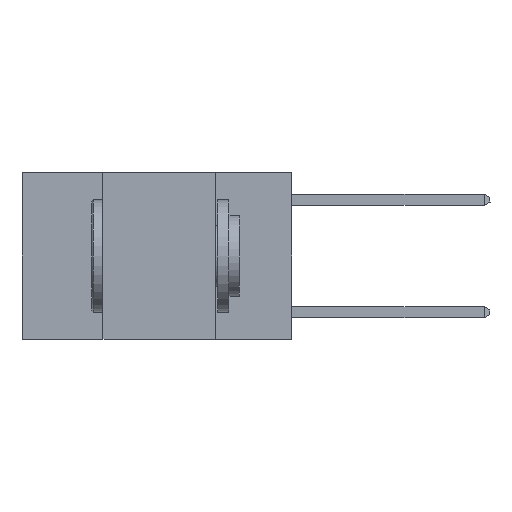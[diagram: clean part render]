
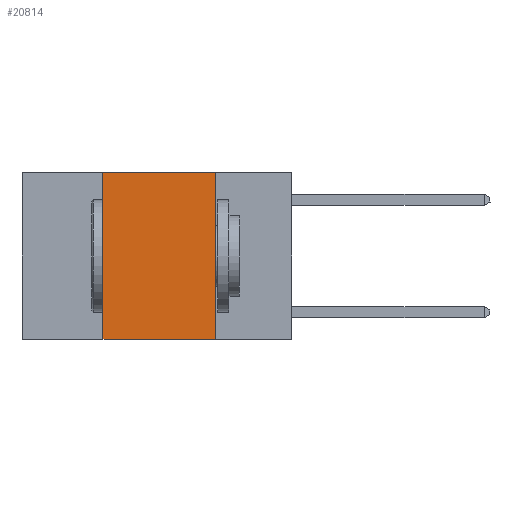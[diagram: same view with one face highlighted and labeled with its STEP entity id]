
A CAD part, left-side view. The second image highlights one B-rep face of the part: STEP entity #20814.
In plain terms, the highlighted planar face has unit normal (-1, 0, 0).
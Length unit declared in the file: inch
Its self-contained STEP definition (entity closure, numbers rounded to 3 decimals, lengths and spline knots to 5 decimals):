
#26 = EDGE_LOOP ( 'NONE', ( #18306, #19401, #16853, #20343 ) ) ;
#2577 = PLANE ( 'NONE',  #20135 ) ;
#3623 = EDGE_CURVE ( 'NONE', #7299, #16457, #7238, .T. ) ;
#6611 = CARTESIAN_POINT ( 'NONE',  ( 0., 0.6, -0.37 ) ) ;
#7238 = LINE ( 'NONE', #9795, #25332 ) ;
#7299 = VERTEX_POINT ( 'NONE', #25105 ) ;
#7310 = EDGE_CURVE ( 'NONE', #16457, #23363, #14555, .T. ) ;
#7414 = VECTOR ( 'NONE', #15293, 39.37008 ) ;
#9041 = CARTESIAN_POINT ( 'NONE',  ( 0., 0.17, -0.37 ) ) ;
#9290 = DIRECTION ( 'NONE',  ( 1., 0., 0. ) ) ;
#9795 = CARTESIAN_POINT ( 'NONE',  ( 0., 0.6, 0. ) ) ;
#10997 = CARTESIAN_POINT ( 'NONE',  ( 0., 0.17, 0. ) ) ;
#12418 = CARTESIAN_POINT ( 'NONE',  ( 0., 0.17, 0. ) ) ;
#12852 = DIRECTION ( 'NONE',  ( 0., 0., 1. ) ) ;
#13236 = VECTOR ( 'NONE', #12852, 39.37008 ) ;
#13284 = EDGE_CURVE ( 'NONE', #24612, #23363, #26128, .T. ) ;
#13705 = CARTESIAN_POINT ( 'NONE',  ( 0., 0.6, 0. ) ) ;
#14409 = DIRECTION ( 'NONE',  ( 0., 0., -1. ) ) ;
#14555 = LINE ( 'NONE', #12418, #18821 ) ;
#14986 = LINE ( 'NONE', #23656, #13236 ) ;
#15293 = DIRECTION ( 'NONE',  ( 0., -1., 0. ) ) ;
#16457 = VERTEX_POINT ( 'NONE', #10997 ) ;
#16853 = ORIENTED_EDGE ( 'NONE', *, *, #19331, .F. ) ;
#18306 = ORIENTED_EDGE ( 'NONE', *, *, #7310, .F. ) ;
#18821 = VECTOR ( 'NONE', #14409, 39.37008 ) ;
#19331 = EDGE_CURVE ( 'NONE', #24612, #7299, #14986, .T. ) ;
#19401 = ORIENTED_EDGE ( 'NONE', *, *, #3623, .F. ) ;
#20135 = AXIS2_PLACEMENT_3D ( 'NONE', #13705, #9290, #22108 ) ;
#20199 = DIRECTION ( 'NONE',  ( 0., -1., 0. ) ) ;
#20343 = ORIENTED_EDGE ( 'NONE', *, *, #13284, .T. ) ;
#20814 = ADVANCED_FACE ( 'NONE', ( #26530 ), #2577, .F. ) ;
#22108 = DIRECTION ( 'NONE',  ( 0., 0., -1. ) ) ;
#23363 = VERTEX_POINT ( 'NONE', #9041 ) ;
#23656 = CARTESIAN_POINT ( 'NONE',  ( 0., 0.42, 0. ) ) ;
#24612 = VERTEX_POINT ( 'NONE', #25186 ) ;
#25105 = CARTESIAN_POINT ( 'NONE',  ( 0., 0.42, 0. ) ) ;
#25186 = CARTESIAN_POINT ( 'NONE',  ( 0., 0.42, -0.37 ) ) ;
#25332 = VECTOR ( 'NONE', #20199, 39.37008 ) ;
#26128 = LINE ( 'NONE', #6611, #7414 ) ;
#26530 = FACE_OUTER_BOUND ( 'NONE', #26, .T. ) ;
